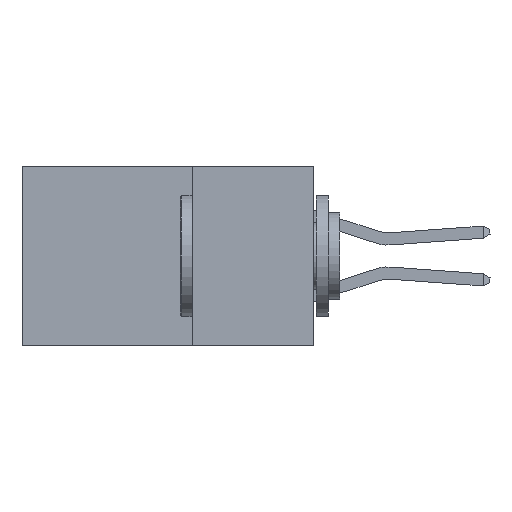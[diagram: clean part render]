
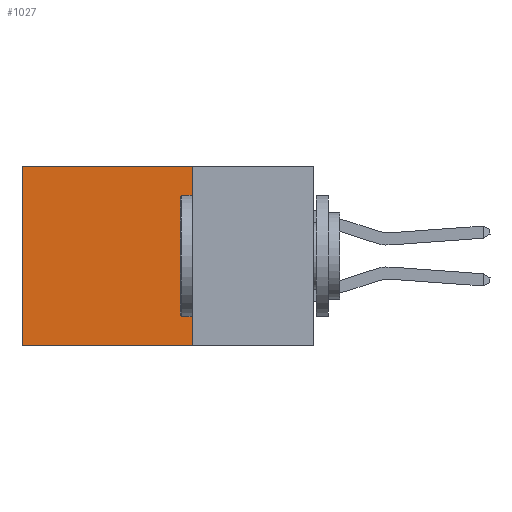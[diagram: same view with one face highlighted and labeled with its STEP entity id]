
A CAD part, left-side view. The second image highlights one B-rep face of the part: STEP entity #1027.
In plain terms, the highlighted planar face has unit normal (-1, 0, 0).
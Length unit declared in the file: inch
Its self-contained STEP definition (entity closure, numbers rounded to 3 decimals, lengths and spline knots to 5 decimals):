
#1012 = VERTEX_POINT ( 'NONE', #10490 ) ;
#1027 = ADVANCED_FACE ( 'NONE', ( #5390 ), #21547, .F. ) ;
#1147 = VECTOR ( 'NONE', #14384, 39.37008 ) ;
#1490 = VERTEX_POINT ( 'NONE', #17825 ) ;
#1945 = VECTOR ( 'NONE', #17578, 39.37008 ) ;
#2054 = CARTESIAN_POINT ( 'NONE',  ( 0.2875, 0.6, 0. ) ) ;
#2861 = CARTESIAN_POINT ( 'NONE',  ( 0.2875, 0.25, 0. ) ) ;
#3215 = AXIS2_PLACEMENT_3D ( 'NONE', #10509, #9634, #9531 ) ;
#4368 = ORIENTED_EDGE ( 'NONE', *, *, #21552, .F. ) ;
#5229 = ORIENTED_EDGE ( 'NONE', *, *, #6300, .T. ) ;
#5390 = FACE_OUTER_BOUND ( 'NONE', #13078, .T. ) ;
#6300 = EDGE_CURVE ( 'NONE', #1012, #6392, #7339, .T. ) ;
#6392 = VERTEX_POINT ( 'NONE', #15419 ) ;
#6726 = LINE ( 'NONE', #15915, #1945 ) ;
#6798 = VECTOR ( 'NONE', #13422, 39.37008 ) ;
#7108 = LINE ( 'NONE', #16999, #12320 ) ;
#7339 = LINE ( 'NONE', #2861, #6798 ) ;
#9531 = DIRECTION ( 'NONE',  ( 0., 0., -1. ) ) ;
#9634 = DIRECTION ( 'NONE',  ( 1., 0., 0. ) ) ;
#10490 = CARTESIAN_POINT ( 'NONE',  ( 0.2875, 0.25, 0. ) ) ;
#10509 = CARTESIAN_POINT ( 'NONE',  ( 0.2875, 0.25, 0. ) ) ;
#10660 = LINE ( 'NONE', #2054, #1147 ) ;
#11530 = EDGE_CURVE ( 'NONE', #6392, #21590, #10660, .T. ) ;
#12320 = VECTOR ( 'NONE', #13683, 39.37008 ) ;
#13078 = EDGE_LOOP ( 'NONE', ( #13780, #4368, #17060, #5229 ) ) ;
#13422 = DIRECTION ( 'NONE',  ( 0., 1., 0. ) ) ;
#13683 = DIRECTION ( 'NONE',  ( 0., 1., 0. ) ) ;
#13780 = ORIENTED_EDGE ( 'NONE', *, *, #11530, .T. ) ;
#14384 = DIRECTION ( 'NONE',  ( 0., 0., -1. ) ) ;
#14590 = EDGE_CURVE ( 'NONE', #1012, #1490, #6726, .T. ) ;
#15419 = CARTESIAN_POINT ( 'NONE',  ( 0.2875, 0.6, 0. ) ) ;
#15915 = CARTESIAN_POINT ( 'NONE',  ( 0.2875, 0.25, 0. ) ) ;
#16999 = CARTESIAN_POINT ( 'NONE',  ( 0.2875, 0.25, -0.37 ) ) ;
#17060 = ORIENTED_EDGE ( 'NONE', *, *, #14590, .F. ) ;
#17578 = DIRECTION ( 'NONE',  ( 0., 0., -1. ) ) ;
#17825 = CARTESIAN_POINT ( 'NONE',  ( 0.2875, 0.25, -0.37 ) ) ;
#21547 = PLANE ( 'NONE',  #3215 ) ;
#21552 = EDGE_CURVE ( 'NONE', #1490, #21590, #7108, .T. ) ;
#21590 = VERTEX_POINT ( 'NONE', #22240 ) ;
#22240 = CARTESIAN_POINT ( 'NONE',  ( 0.2875, 0.6, -0.37 ) ) ;
